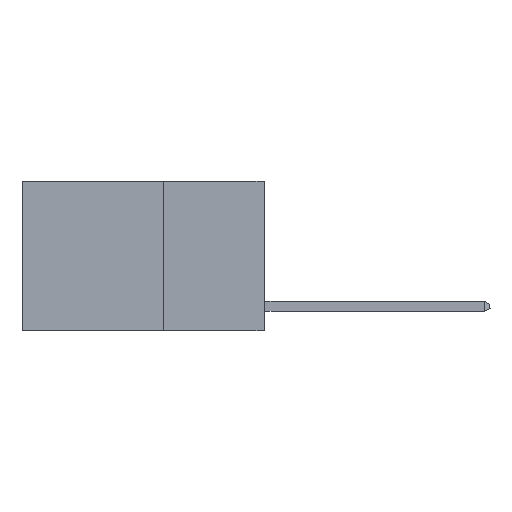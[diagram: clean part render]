
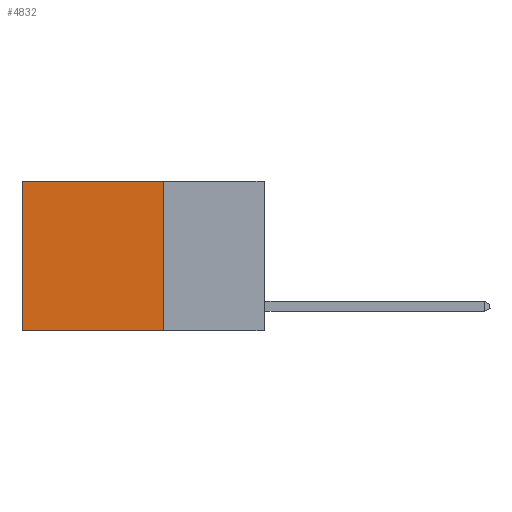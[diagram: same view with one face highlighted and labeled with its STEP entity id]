
A CAD part, left-side view. The second image highlights one B-rep face of the part: STEP entity #4832.
In plain terms, the highlighted planar face has unit normal (-1, 0, 0).
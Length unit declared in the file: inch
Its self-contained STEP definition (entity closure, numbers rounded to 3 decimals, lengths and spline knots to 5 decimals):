
#172 = CARTESIAN_POINT ( 'NONE',  ( 0.2625, 0.25, 0. ) ) ;
#304 = CARTESIAN_POINT ( 'NONE',  ( 0.2625, 0.25, 0. ) ) ;
#980 = PLANE ( 'NONE',  #8155 ) ;
#1009 = CARTESIAN_POINT ( 'NONE',  ( 0.2625, 0.25, -0.37 ) ) ;
#1499 = EDGE_CURVE ( 'NONE', #5238, #5569, #8413, .T. ) ;
#2346 = VECTOR ( 'NONE', #9501, 39.37008 ) ;
#2517 = ORIENTED_EDGE ( 'NONE', *, *, #9410, .F. ) ;
#2565 = DIRECTION ( 'NONE',  ( 0., 1., 0. ) ) ;
#2713 = DIRECTION ( 'NONE',  ( 0., 0., -1. ) ) ;
#3545 = CARTESIAN_POINT ( 'NONE',  ( 0.2625, 0.6, 0. ) ) ;
#3756 = CARTESIAN_POINT ( 'NONE',  ( 0.2625, 0.6, -0.37 ) ) ;
#4065 = ORIENTED_EDGE ( 'NONE', *, *, #1499, .F. ) ;
#4318 = ORIENTED_EDGE ( 'NONE', *, *, #10079, .T. ) ;
#4800 = VECTOR ( 'NONE', #2713, 39.37008 ) ;
#4832 = ADVANCED_FACE ( 'NONE', ( #8285 ), #980, .F. ) ;
#4865 = LINE ( 'NONE', #1009, #10398 ) ;
#4896 = ORIENTED_EDGE ( 'NONE', *, *, #4919, .T. ) ;
#4913 = VERTEX_POINT ( 'NONE', #3756 ) ;
#4915 = VERTEX_POINT ( 'NONE', #6059 ) ;
#4919 = EDGE_CURVE ( 'NONE', #4915, #4913, #7040, .T. ) ;
#5106 = CARTESIAN_POINT ( 'NONE',  ( 0.2625, 0.25, 0. ) ) ;
#5238 = VERTEX_POINT ( 'NONE', #304 ) ;
#5462 = CARTESIAN_POINT ( 'NONE',  ( 0.2625, 0.25, -0.37 ) ) ;
#5569 = VERTEX_POINT ( 'NONE', #5462 ) ;
#5803 = DIRECTION ( 'NONE',  ( 1., 0., 0. ) ) ;
#6059 = CARTESIAN_POINT ( 'NONE',  ( 0.2625, 0.6, 0. ) ) ;
#7007 = VECTOR ( 'NONE', #7104, 39.37008 ) ;
#7040 = LINE ( 'NONE', #3545, #2346 ) ;
#7104 = DIRECTION ( 'NONE',  ( 0., 1., 0. ) ) ;
#8155 = AXIS2_PLACEMENT_3D ( 'NONE', #5106, #5803, #8387 ) ;
#8285 = FACE_OUTER_BOUND ( 'NONE', #8721, .T. ) ;
#8387 = DIRECTION ( 'NONE',  ( 0., 0., -1. ) ) ;
#8413 = LINE ( 'NONE', #172, #4800 ) ;
#8721 = EDGE_LOOP ( 'NONE', ( #4896, #2517, #4065, #4318 ) ) ;
#9410 = EDGE_CURVE ( 'NONE', #5569, #4913, #4865, .T. ) ;
#9466 = CARTESIAN_POINT ( 'NONE',  ( 0.2625, 0.25, 0. ) ) ;
#9501 = DIRECTION ( 'NONE',  ( 0., 0., -1. ) ) ;
#10079 = EDGE_CURVE ( 'NONE', #5238, #4915, #10460, .T. ) ;
#10398 = VECTOR ( 'NONE', #2565, 39.37008 ) ;
#10460 = LINE ( 'NONE', #9466, #7007 ) ;
